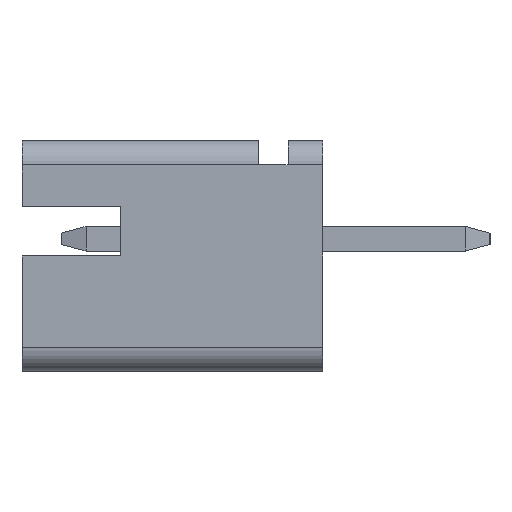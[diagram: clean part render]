
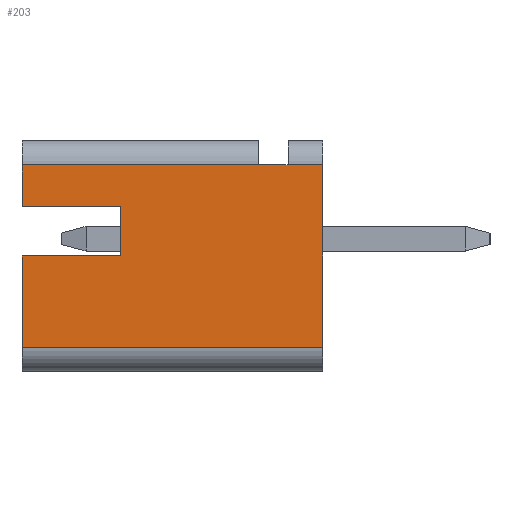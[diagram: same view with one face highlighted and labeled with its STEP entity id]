
A CAD part, left-side view. The second image highlights one B-rep face of the part: STEP entity #203.
In plain terms, the highlighted planar face has unit normal (-1, 0, 0).
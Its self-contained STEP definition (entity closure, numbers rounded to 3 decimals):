
#5 = DIRECTION ( 'NONE',  ( 1., 0., 0. ) ) ;
#16 = CARTESIAN_POINT ( 'NONE',  ( -2., 1.3, 1.5 ) ) ;
#42 = DIRECTION ( 'NONE',  ( 0., -1., 0. ) ) ;
#60 = EDGE_LOOP ( 'NONE', ( #3261, #2493, #4720, #165, #4897, #737, #488, #1200, #3285, #3494 ) ) ;
#69 = EDGE_CURVE ( 'NONE', #1109, #1442, #1794, .T. ) ;
#97 = LINE ( 'NONE', #472, #4291 ) ;
#165 = ORIENTED_EDGE ( 'NONE', *, *, #1435, .T. ) ;
#203 = ADVANCED_FACE ( 'NONE', ( #3064 ), #4935, .F. ) ;
#300 = CARTESIAN_POINT ( 'NONE',  ( -2., 4.1, 0.65 ) ) ;
#472 = CARTESIAN_POINT ( 'NONE',  ( -2., 0., 1.5 ) ) ;
#488 = ORIENTED_EDGE ( 'NONE', *, *, #1025, .F. ) ;
#549 = CARTESIAN_POINT ( 'NONE',  ( -2., 6.1, -0.35 ) ) ;
#590 = EDGE_CURVE ( 'NONE', #2233, #1109, #2290, .T. ) ;
#688 = LINE ( 'NONE', #3362, #1177 ) ;
#737 = ORIENTED_EDGE ( 'NONE', *, *, #3412, .T. ) ;
#846 = CARTESIAN_POINT ( 'NONE',  ( -2., 6.1, -2.2 ) ) ;
#853 = DIRECTION ( 'NONE',  ( 0., 0., -1. ) ) ;
#938 = LINE ( 'NONE', #989, #3096 ) ;
#968 = AXIS2_PLACEMENT_3D ( 'NONE', #3039, #5, #853 ) ;
#989 = CARTESIAN_POINT ( 'NONE',  ( -2., 0., -2.2 ) ) ;
#992 = VECTOR ( 'NONE', #4737, 1000. ) ;
#996 = EDGE_CURVE ( 'NONE', #4348, #3840, #1504, .T. ) ;
#1025 = EDGE_CURVE ( 'NONE', #4148, #4428, #3828, .T. ) ;
#1109 = VERTEX_POINT ( 'NONE', #4325 ) ;
#1177 = VECTOR ( 'NONE', #1321, 1000. ) ;
#1200 = ORIENTED_EDGE ( 'NONE', *, *, #1428, .F. ) ;
#1286 = CARTESIAN_POINT ( 'NONE',  ( -2., 0., -2.2 ) ) ;
#1321 = DIRECTION ( 'NONE',  ( 0., 1., 0. ) ) ;
#1428 = EDGE_CURVE ( 'NONE', #1442, #4148, #3282, .T. ) ;
#1435 = EDGE_CURVE ( 'NONE', #1569, #3840, #688, .T. ) ;
#1442 = VERTEX_POINT ( 'NONE', #300 ) ;
#1486 = DIRECTION ( 'NONE',  ( 0., -1., 0. ) ) ;
#1504 = LINE ( 'NONE', #16, #2981 ) ;
#1569 = VERTEX_POINT ( 'NONE', #2066 ) ;
#1578 = EDGE_CURVE ( 'NONE', #3471, #3369, #938, .T. ) ;
#1579 = VECTOR ( 'NONE', #4489, 1000. ) ;
#1596 = CARTESIAN_POINT ( 'NONE',  ( -2., 6.1, 1.5 ) ) ;
#1794 = LINE ( 'NONE', #2640, #2444 ) ;
#1828 = CARTESIAN_POINT ( 'NONE',  ( -2., 1.3, 1.5 ) ) ;
#1912 = DIRECTION ( 'NONE',  ( 0., -1., 0. ) ) ;
#1930 = CARTESIAN_POINT ( 'NONE',  ( -2., 6.1, -0.35 ) ) ;
#2066 = CARTESIAN_POINT ( 'NONE',  ( -2., 0., 1.5 ) ) ;
#2160 = CARTESIAN_POINT ( 'NONE',  ( -2., 0., 2. ) ) ;
#2225 = CARTESIAN_POINT ( 'NONE',  ( -2., 6.1, 0.65 ) ) ;
#2233 = VERTEX_POINT ( 'NONE', #1930 ) ;
#2290 = LINE ( 'NONE', #3810, #4102 ) ;
#2379 = VECTOR ( 'NONE', #4479, 1000. ) ;
#2444 = VECTOR ( 'NONE', #3320, 1000. ) ;
#2493 = ORIENTED_EDGE ( 'NONE', *, *, #1578, .T. ) ;
#2640 = CARTESIAN_POINT ( 'NONE',  ( -2., 4.1, 0.65 ) ) ;
#2728 = CARTESIAN_POINT ( 'NONE',  ( -2., 6.1, 2. ) ) ;
#2836 = DIRECTION ( 'NONE',  ( 0., 1., 0. ) ) ;
#2981 = VECTOR ( 'NONE', #42, 1000. ) ;
#3039 = CARTESIAN_POINT ( 'NONE',  ( -2., 0., 0. ) ) ;
#3064 = FACE_OUTER_BOUND ( 'NONE', #60, .T. ) ;
#3096 = VECTOR ( 'NONE', #1486, 1000. ) ;
#3105 = EDGE_CURVE ( 'NONE', #1569, #3369, #4041, .T. ) ;
#3261 = ORIENTED_EDGE ( 'NONE', *, *, #3480, .F. ) ;
#3282 = LINE ( 'NONE', #2225, #1579 ) ;
#3285 = ORIENTED_EDGE ( 'NONE', *, *, #69, .F. ) ;
#3320 = DIRECTION ( 'NONE',  ( 0., 0., 1. ) ) ;
#3362 = CARTESIAN_POINT ( 'NONE',  ( -2., 0., 1.5 ) ) ;
#3369 = VERTEX_POINT ( 'NONE', #1286 ) ;
#3412 = EDGE_CURVE ( 'NONE', #4348, #4428, #97, .T. ) ;
#3471 = VERTEX_POINT ( 'NONE', #846 ) ;
#3480 = EDGE_CURVE ( 'NONE', #3471, #2233, #3607, .T. ) ;
#3494 = ORIENTED_EDGE ( 'NONE', *, *, #590, .F. ) ;
#3579 = CARTESIAN_POINT ( 'NONE',  ( -2., 6.1, 0.65 ) ) ;
#3607 = LINE ( 'NONE', #549, #992 ) ;
#3810 = CARTESIAN_POINT ( 'NONE',  ( -2., 6.1, -0.35 ) ) ;
#3828 = LINE ( 'NONE', #2728, #4023 ) ;
#3840 = VERTEX_POINT ( 'NONE', #4159 ) ;
#4023 = VECTOR ( 'NONE', #4250, 1000. ) ;
#4041 = LINE ( 'NONE', #2160, #2379 ) ;
#4102 = VECTOR ( 'NONE', #1912, 1000. ) ;
#4148 = VERTEX_POINT ( 'NONE', #3579 ) ;
#4159 = CARTESIAN_POINT ( 'NONE',  ( -2., 0.7, 1.5 ) ) ;
#4250 = DIRECTION ( 'NONE',  ( 0., 0., 1. ) ) ;
#4291 = VECTOR ( 'NONE', #2836, 1000. ) ;
#4325 = CARTESIAN_POINT ( 'NONE',  ( -2., 4.1, -0.35 ) ) ;
#4348 = VERTEX_POINT ( 'NONE', #1828 ) ;
#4428 = VERTEX_POINT ( 'NONE', #1596 ) ;
#4479 = DIRECTION ( 'NONE',  ( 0., 0., -1. ) ) ;
#4489 = DIRECTION ( 'NONE',  ( 0., 1., 0. ) ) ;
#4720 = ORIENTED_EDGE ( 'NONE', *, *, #3105, .F. ) ;
#4737 = DIRECTION ( 'NONE',  ( 0., 0., 1. ) ) ;
#4897 = ORIENTED_EDGE ( 'NONE', *, *, #996, .F. ) ;
#4935 = PLANE ( 'NONE',  #968 ) ;
